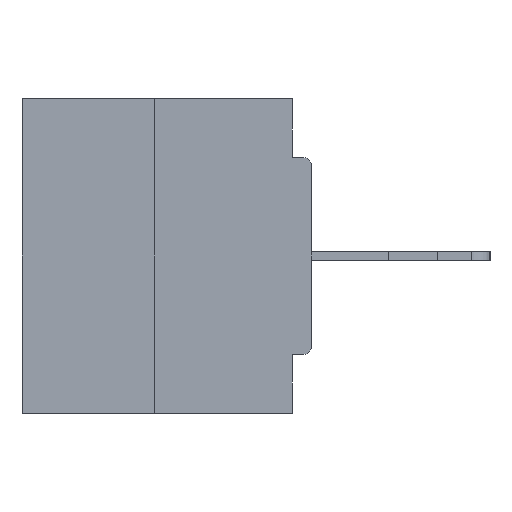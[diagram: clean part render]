
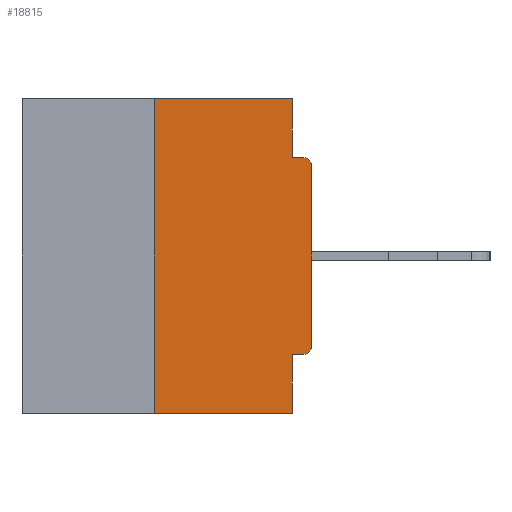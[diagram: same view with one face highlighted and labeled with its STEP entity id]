
A CAD part, left-side view. The second image highlights one B-rep face of the part: STEP entity #18815.
In plain terms, the highlighted planar face has unit normal (-1, 0, 0).
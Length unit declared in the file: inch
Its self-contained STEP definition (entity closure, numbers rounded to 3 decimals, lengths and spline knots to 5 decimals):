
#37 = CARTESIAN_POINT ( 'NONE',  ( 0., 0.031, -0.4065 ) ) ;
#205 = DIRECTION ( 'NONE',  ( 0., 0., -1. ) ) ;
#2656 = VECTOR ( 'NONE', #36051, 39.37008 ) ;
#2688 = CARTESIAN_POINT ( 'NONE',  ( 0., 0.25, 0. ) ) ;
#2752 = CIRCLE ( 'NONE', #24456, 0.015 ) ;
#3883 = ORIENTED_EDGE ( 'NONE', *, *, #16030, .F. ) ;
#4311 = CARTESIAN_POINT ( 'NONE',  ( 0., 0.031, 0. ) ) ;
#4714 = LINE ( 'NONE', #8289, #14309 ) ;
#5640 = DIRECTION ( 'NONE',  ( -1., 0., 0. ) ) ;
#5775 = LINE ( 'NONE', #25983, #20669 ) ;
#5886 = ORIENTED_EDGE ( 'NONE', *, *, #13763, .T. ) ;
#5887 = PLANE ( 'NONE',  #15209 ) ;
#6404 = DIRECTION ( 'NONE',  ( 0., 0., -1. ) ) ;
#6685 = VERTEX_POINT ( 'NONE', #29111 ) ;
#7231 = CARTESIAN_POINT ( 'NONE',  ( 0., 0.015, -0.0935 ) ) ;
#8289 = CARTESIAN_POINT ( 'NONE',  ( 0., 0., -0.0935 ) ) ;
#8313 = CARTESIAN_POINT ( 'NONE',  ( 0., 0.46, 0. ) ) ;
#8314 = LINE ( 'NONE', #13981, #23836 ) ;
#9145 = EDGE_CURVE ( 'NONE', #6685, #15251, #8314, .T. ) ;
#9471 = CARTESIAN_POINT ( 'NONE',  ( 0., 0.015, -0.3915 ) ) ;
#9556 = AXIS2_PLACEMENT_3D ( 'NONE', #9471, #23436, #205 ) ;
#9632 = CARTESIAN_POINT ( 'NONE',  ( 0., 0., 0. ) ) ;
#10736 = ORIENTED_EDGE ( 'NONE', *, *, #30686, .F. ) ;
#11380 = DIRECTION ( 'NONE',  ( 0., 0., 1. ) ) ;
#11802 = CARTESIAN_POINT ( 'NONE',  ( 0., 0.031, -0.0935 ) ) ;
#11840 = VERTEX_POINT ( 'NONE', #27423 ) ;
#12798 = ORIENTED_EDGE ( 'NONE', *, *, #20629, .F. ) ;
#13763 = EDGE_CURVE ( 'NONE', #17500, #29009, #14363, .T. ) ;
#13981 = CARTESIAN_POINT ( 'NONE',  ( 0., 0.46, -0.5 ) ) ;
#14112 = EDGE_CURVE ( 'NONE', #34042, #32936, #4714, .T. ) ;
#14129 = ORIENTED_EDGE ( 'NONE', *, *, #14112, .F. ) ;
#14309 = VECTOR ( 'NONE', #34180, 39.37008 ) ;
#14363 = CIRCLE ( 'NONE', #9556, 0.015 ) ;
#14664 = DIRECTION ( 'NONE',  ( 0., 1., 0. ) ) ;
#15188 = VERTEX_POINT ( 'NONE', #18706 ) ;
#15209 = AXIS2_PLACEMENT_3D ( 'NONE', #31585, #23454, #25905 ) ;
#15251 = VERTEX_POINT ( 'NONE', #33444 ) ;
#15301 = LINE ( 'NONE', #9632, #2656 ) ;
#16030 = EDGE_CURVE ( 'NONE', #20037, #15251, #18616, .T. ) ;
#17500 = VERTEX_POINT ( 'NONE', #17599 ) ;
#17570 = ORIENTED_EDGE ( 'NONE', *, *, #30484, .T. ) ;
#17599 = CARTESIAN_POINT ( 'NONE',  ( 0., 0.015, -0.4065 ) ) ;
#18301 = LINE ( 'NONE', #4311, #36542 ) ;
#18616 = LINE ( 'NONE', #20904, #22860 ) ;
#18706 = CARTESIAN_POINT ( 'NONE',  ( 0., 0.25, 0. ) ) ;
#18815 = ADVANCED_FACE ( 'NONE', ( #31956 ), #5887, .F. ) ;
#20037 = VERTEX_POINT ( 'NONE', #37 ) ;
#20629 = EDGE_CURVE ( 'NONE', #6685, #15188, #28555, .T. ) ;
#20669 = VECTOR ( 'NONE', #14664, 39.37008 ) ;
#20904 = CARTESIAN_POINT ( 'NONE',  ( 0., 0.031, -0.5 ) ) ;
#21757 = CARTESIAN_POINT ( 'NONE',  ( 0., 0., -0.1085 ) ) ;
#22174 = EDGE_CURVE ( 'NONE', #15188, #11840, #30800, .T. ) ;
#22471 = EDGE_CURVE ( 'NONE', #29009, #25237, #15301, .T. ) ;
#22860 = VECTOR ( 'NONE', #32806, 39.37008 ) ;
#23131 = VECTOR ( 'NONE', #31172, 39.37008 ) ;
#23436 = DIRECTION ( 'NONE',  ( -1., 0., 0. ) ) ;
#23454 = DIRECTION ( 'NONE',  ( 1., 0., 0. ) ) ;
#23788 = DIRECTION ( 'NONE',  ( 0., 0., -1. ) ) ;
#23836 = VECTOR ( 'NONE', #25311, 39.37008 ) ;
#24456 = AXIS2_PLACEMENT_3D ( 'NONE', #34749, #5640, #6404 ) ;
#24840 = VECTOR ( 'NONE', #11380, 39.37008 ) ;
#25237 = VERTEX_POINT ( 'NONE', #21757 ) ;
#25311 = DIRECTION ( 'NONE',  ( 0., -1., 0. ) ) ;
#25905 = DIRECTION ( 'NONE',  ( 0., 0., -1. ) ) ;
#25983 = CARTESIAN_POINT ( 'NONE',  ( 0., 0., -0.4065 ) ) ;
#27423 = CARTESIAN_POINT ( 'NONE',  ( 0., 0.031, 0. ) ) ;
#27544 = EDGE_CURVE ( 'NONE', #17500, #20037, #5775, .T. ) ;
#27966 = ORIENTED_EDGE ( 'NONE', *, *, #9145, .T. ) ;
#28555 = LINE ( 'NONE', #2688, #24840 ) ;
#29009 = VERTEX_POINT ( 'NONE', #32512 ) ;
#29111 = CARTESIAN_POINT ( 'NONE',  ( 0., 0.25, -0.5 ) ) ;
#30484 = EDGE_CURVE ( 'NONE', #25237, #32936, #2752, .T. ) ;
#30686 = EDGE_CURVE ( 'NONE', #11840, #34042, #18301, .T. ) ;
#30800 = LINE ( 'NONE', #8313, #23131 ) ;
#31099 = ORIENTED_EDGE ( 'NONE', *, *, #22471, .T. ) ;
#31172 = DIRECTION ( 'NONE',  ( 0., -1., 0. ) ) ;
#31294 = ORIENTED_EDGE ( 'NONE', *, *, #27544, .F. ) ;
#31585 = CARTESIAN_POINT ( 'NONE',  ( 0., 0.46, 0. ) ) ;
#31900 = EDGE_LOOP ( 'NONE', ( #37095, #12798, #27966, #3883, #31294, #5886, #31099, #17570, #14129, #10736 ) ) ;
#31956 = FACE_OUTER_BOUND ( 'NONE', #31900, .T. ) ;
#32512 = CARTESIAN_POINT ( 'NONE',  ( 0., 0., -0.3915 ) ) ;
#32806 = DIRECTION ( 'NONE',  ( 0., 0., -1. ) ) ;
#32936 = VERTEX_POINT ( 'NONE', #7231 ) ;
#33444 = CARTESIAN_POINT ( 'NONE',  ( 0., 0.031, -0.5 ) ) ;
#34042 = VERTEX_POINT ( 'NONE', #11802 ) ;
#34180 = DIRECTION ( 'NONE',  ( 0., -1., 0. ) ) ;
#34749 = CARTESIAN_POINT ( 'NONE',  ( 0., 0.015, -0.1085 ) ) ;
#36051 = DIRECTION ( 'NONE',  ( 0., 0., 1. ) ) ;
#36542 = VECTOR ( 'NONE', #23788, 39.37008 ) ;
#37095 = ORIENTED_EDGE ( 'NONE', *, *, #22174, .F. ) ;
